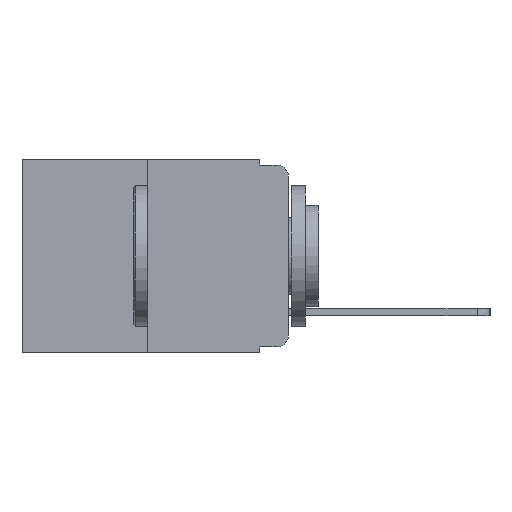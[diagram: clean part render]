
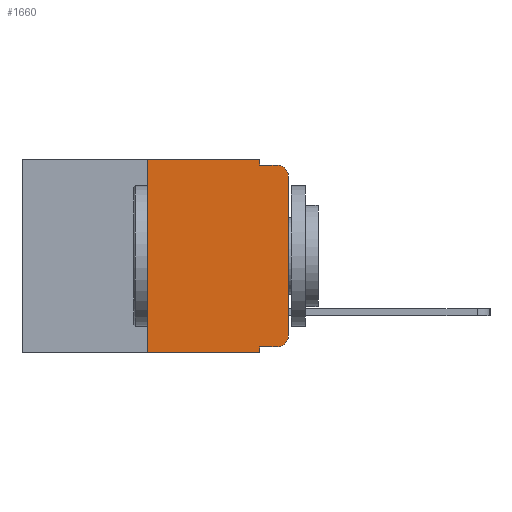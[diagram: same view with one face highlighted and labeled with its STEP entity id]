
A CAD part, left-side view. The second image highlights one B-rep face of the part: STEP entity #1660.
In plain terms, the highlighted planar face has unit normal (-1, 0, 0).
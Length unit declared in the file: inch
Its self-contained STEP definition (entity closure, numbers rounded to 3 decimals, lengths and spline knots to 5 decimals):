
#67 = VERTEX_POINT ( 'NONE', #3621 ) ;
#94 = CARTESIAN_POINT ( 'NONE',  ( 0., 0.051, 0. ) ) ;
#362 = VERTEX_POINT ( 'NONE', #9676 ) ;
#546 = AXIS2_PLACEMENT_3D ( 'NONE', #1407, #8310, #2459 ) ;
#571 = VERTEX_POINT ( 'NONE', #7963 ) ;
#688 = AXIS2_PLACEMENT_3D ( 'NONE', #8008, #2134, #8966 ) ;
#922 = CIRCLE ( 'NONE', #546, 0.02 ) ;
#1198 = DIRECTION ( 'NONE',  ( 0., 0., 1. ) ) ;
#1407 = CARTESIAN_POINT ( 'NONE',  ( 0., 0.02, -0.313 ) ) ;
#1476 = VECTOR ( 'NONE', #8802, 39.37008 ) ;
#1645 = LINE ( 'NONE', #94, #6965 ) ;
#1660 = ADVANCED_FACE ( 'NONE', ( #7989 ), #2235, .F. ) ;
#2134 = DIRECTION ( 'NONE',  ( -1., 0., 0. ) ) ;
#2235 = PLANE ( 'NONE',  #4674 ) ;
#2288 = VECTOR ( 'NONE', #10704, 39.37008 ) ;
#2459 = DIRECTION ( 'NONE',  ( 0., 0., -1. ) ) ;
#2530 = DIRECTION ( 'NONE',  ( 1., 0., 0. ) ) ;
#2633 = LINE ( 'NONE', #4416, #7545 ) ;
#2908 = DIRECTION ( 'NONE',  ( 0., -1., 0. ) ) ;
#3146 = DIRECTION ( 'NONE',  ( 0., -1., 0. ) ) ;
#3199 = VERTEX_POINT ( 'NONE', #8176 ) ;
#3223 = DIRECTION ( 'NONE',  ( 0., 0., -1. ) ) ;
#3333 = VERTEX_POINT ( 'NONE', #8131 ) ;
#3506 = LINE ( 'NONE', #11855, #8255 ) ;
#3621 = CARTESIAN_POINT ( 'NONE',  ( 0., 0.051, -0.01 ) ) ;
#3879 = VECTOR ( 'NONE', #11756, 39.37008 ) ;
#4294 = CARTESIAN_POINT ( 'NONE',  ( 0., 0.02, -0.01 ) ) ;
#4416 = CARTESIAN_POINT ( 'NONE',  ( 0., 0.051, -0.01 ) ) ;
#4674 = AXIS2_PLACEMENT_3D ( 'NONE', #8706, #2530, #3223 ) ;
#4725 = EDGE_CURVE ( 'NONE', #571, #3333, #3506, .T. ) ;
#4891 = VECTOR ( 'NONE', #1198, 39.37008 ) ;
#5385 = DIRECTION ( 'NONE',  ( 0., -1., 0. ) ) ;
#5579 = CARTESIAN_POINT ( 'NONE',  ( 0., 0.051, -0.333 ) ) ;
#5713 = CIRCLE ( 'NONE', #688, 0.02 ) ;
#5923 = CARTESIAN_POINT ( 'NONE',  ( 0., 0.473, -0.343 ) ) ;
#6394 = DIRECTION ( 'NONE',  ( 0., 0., -1. ) ) ;
#6585 = VERTEX_POINT ( 'NONE', #4294 ) ;
#6611 = CARTESIAN_POINT ( 'NONE',  ( 0., 0.02, -0.333 ) ) ;
#6631 = VECTOR ( 'NONE', #2908, 39.37008 ) ;
#6905 = LINE ( 'NONE', #5923, #6631 ) ;
#6965 = VECTOR ( 'NONE', #6394, 39.37008 ) ;
#7281 = EDGE_LOOP ( 'NONE', ( #8419, #9007, #9241, #9581, #9708, #9722, #10303, #10676, #10715, #10908 ) ) ;
#7545 = VECTOR ( 'NONE', #5385, 39.37008 ) ;
#7817 = VERTEX_POINT ( 'NONE', #9820 ) ;
#7850 = CARTESIAN_POINT ( 'NONE',  ( 0., 0., 0. ) ) ;
#7963 = CARTESIAN_POINT ( 'NONE',  ( 0., 0.25, 0. ) ) ;
#7989 = FACE_OUTER_BOUND ( 'NONE', #7281, .T. ) ;
#8008 = CARTESIAN_POINT ( 'NONE',  ( 0., 0.02, -0.03 ) ) ;
#8088 = VERTEX_POINT ( 'NONE', #6611 ) ;
#8131 = CARTESIAN_POINT ( 'NONE',  ( 0., 0.051, 0. ) ) ;
#8176 = CARTESIAN_POINT ( 'NONE',  ( 0., 0.051, -0.333 ) ) ;
#8255 = VECTOR ( 'NONE', #3146, 39.37008 ) ;
#8310 = DIRECTION ( 'NONE',  ( -1., 0., 0. ) ) ;
#8371 = VERTEX_POINT ( 'NONE', #8981 ) ;
#8419 = ORIENTED_EDGE ( 'NONE', *, *, #11222, .T. ) ;
#8706 = CARTESIAN_POINT ( 'NONE',  ( 0., 0.473, 0. ) ) ;
#8802 = DIRECTION ( 'NONE',  ( 0., 0., 1. ) ) ;
#8812 = EDGE_CURVE ( 'NONE', #7817, #9670, #6905, .T. ) ;
#8966 = DIRECTION ( 'NONE',  ( 0., 0., -1. ) ) ;
#8981 = CARTESIAN_POINT ( 'NONE',  ( 0., 0., -0.313 ) ) ;
#9007 = ORIENTED_EDGE ( 'NONE', *, *, #11321, .T. ) ;
#9241 = ORIENTED_EDGE ( 'NONE', *, *, #11368, .F. ) ;
#9265 = LINE ( 'NONE', #7850, #1476 ) ;
#9581 = ORIENTED_EDGE ( 'NONE', *, *, #11370, .F. ) ;
#9670 = VERTEX_POINT ( 'NONE', #12244 ) ;
#9676 = CARTESIAN_POINT ( 'NONE',  ( 0., 0., -0.03 ) ) ;
#9708 = ORIENTED_EDGE ( 'NONE', *, *, #4725, .F. ) ;
#9722 = ORIENTED_EDGE ( 'NONE', *, *, #11384, .F. ) ;
#9820 = CARTESIAN_POINT ( 'NONE',  ( 0., 0.25, -0.343 ) ) ;
#9911 = CARTESIAN_POINT ( 'NONE',  ( 0., 0.051, 0. ) ) ;
#9938 = LINE ( 'NONE', #9911, #2288 ) ;
#10303 = ORIENTED_EDGE ( 'NONE', *, *, #8812, .T. ) ;
#10608 = CARTESIAN_POINT ( 'NONE',  ( 0., 0.25, 0. ) ) ;
#10676 = ORIENTED_EDGE ( 'NONE', *, *, #11428, .F. ) ;
#10704 = DIRECTION ( 'NONE',  ( 0., 0., -1. ) ) ;
#10715 = ORIENTED_EDGE ( 'NONE', *, *, #11466, .T. ) ;
#10908 = ORIENTED_EDGE ( 'NONE', *, *, #11468, .T. ) ;
#11084 = LINE ( 'NONE', #5579, #3879 ) ;
#11222 = EDGE_CURVE ( 'NONE', #8371, #362, #9265, .T. ) ;
#11321 = EDGE_CURVE ( 'NONE', #362, #6585, #5713, .T. ) ;
#11368 = EDGE_CURVE ( 'NONE', #67, #6585, #2633, .T. ) ;
#11370 = EDGE_CURVE ( 'NONE', #3333, #67, #9938, .T. ) ;
#11384 = EDGE_CURVE ( 'NONE', #7817, #571, #11926, .T. ) ;
#11428 = EDGE_CURVE ( 'NONE', #3199, #9670, #1645, .T. ) ;
#11466 = EDGE_CURVE ( 'NONE', #3199, #8088, #11084, .T. ) ;
#11468 = EDGE_CURVE ( 'NONE', #8088, #8371, #922, .T. ) ;
#11756 = DIRECTION ( 'NONE',  ( 0., -1., 0. ) ) ;
#11855 = CARTESIAN_POINT ( 'NONE',  ( 0., 0.473, 0. ) ) ;
#11926 = LINE ( 'NONE', #10608, #4891 ) ;
#12244 = CARTESIAN_POINT ( 'NONE',  ( 0., 0.051, -0.343 ) ) ;
